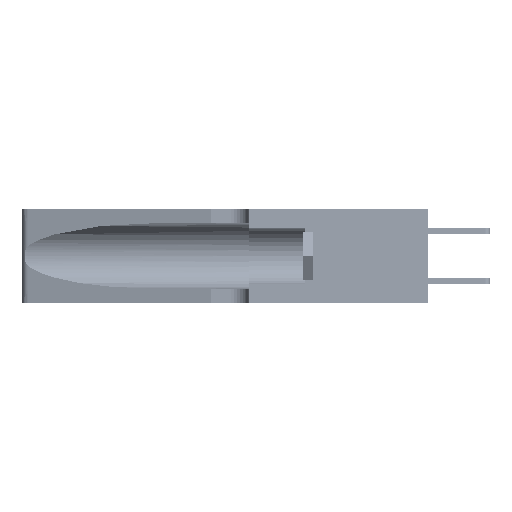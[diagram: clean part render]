
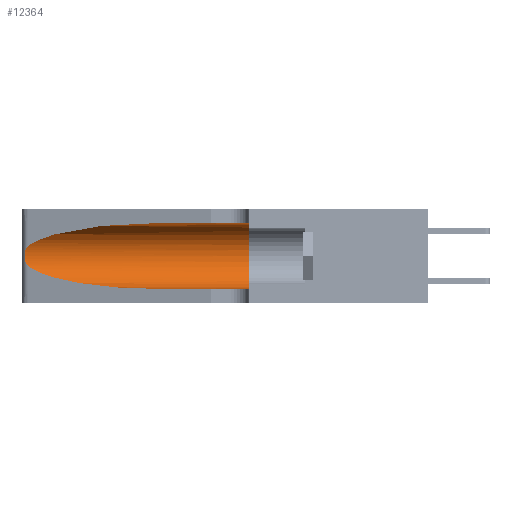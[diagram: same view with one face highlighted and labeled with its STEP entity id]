
A CAD part, left-side view. The second image highlights one B-rep face of the part: STEP entity #12364.
In plain terms, the highlighted cylindrical face has radius 3.308 mm (diameter 6.617 mm), a partial arc.
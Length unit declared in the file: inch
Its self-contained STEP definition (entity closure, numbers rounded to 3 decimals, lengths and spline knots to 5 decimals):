
#735 = CARTESIAN_POINT ( 'NONE',  ( 0.25856, 1.23593, 0.16098 ) ) ;
#1592 = CARTESIAN_POINT ( 'NONE',  ( 0.25487, 1.22718, 0.22369 ) ) ;
#2863 =( BOUNDED_CURVE ( )  B_SPLINE_CURVE ( 3, ( #27474, #7144, #24797, #3694 ),
 .UNSPECIFIED., .F., .F. ) 
 B_SPLINE_CURVE_WITH_KNOTS ( ( 4, 4 ),
 ( 3.44316, 4.71239 ),
 .UNSPECIFIED. ) 
 CURVE ( )  GEOMETRIC_REPRESENTATION_ITEM ( )  RATIONAL_B_SPLINE_CURVE ( ( 1., 0.87, 0.87, 1. ) ) 
 REPRESENTATION_ITEM ( '' )  );
#3694 = CARTESIAN_POINT ( 'NONE',  ( 0.1305, 0.72297, 0.05475 ) ) ;
#3899 = ORIENTED_EDGE ( 'NONE', *, *, #13138, .T. ) ;
#4337 = CARTESIAN_POINT ( 'NONE',  ( 0.1305, 0.35, 0.31525 ) ) ;
#5065 = ORIENTED_EDGE ( 'NONE', *, *, #23339, .T. ) ;
#6265 = DIRECTION ( 'NONE',  ( 0., -1., 0. ) ) ;
#7144 = CARTESIAN_POINT ( 'NONE',  ( 0.2373, 1.15595, 0.08982 ) ) ;
#7562 = DIRECTION ( 'NONE',  ( 0., 0., 1. ) ) ;
#8135 = FACE_OUTER_BOUND ( 'NONE', #32251, .T. ) ;
#8551 =( BOUNDED_CURVE ( )  B_SPLINE_CURVE ( 3, ( #12194, #26577, #44191, #1592 ),
 .UNSPECIFIED., .F., .F. ) 
 B_SPLINE_CURVE_WITH_KNOTS ( ( 4, 4 ),
 ( 1.5708, 2.84003 ),
 .UNSPECIFIED. ) 
 CURVE ( )  GEOMETRIC_REPRESENTATION_ITEM ( )  RATIONAL_B_SPLINE_CURVE ( ( 1., 0.87, 0.87, 1. ) ) 
 REPRESENTATION_ITEM ( '' )  );
#8889 = ORIENTED_EDGE ( 'NONE', *, *, #24045, .T. ) ;
#8992 = VERTEX_POINT ( 'NONE', #41970 ) ;
#9251 = VERTEX_POINT ( 'NONE', #41409 ) ;
#9920 = EDGE_CURVE ( 'NONE', #25475, #9251, #26015, .T. ) ;
#10131 = CARTESIAN_POINT ( 'NONE',  ( 0.1305, 1.61858, 0.05475 ) ) ;
#10462 = DIRECTION ( 'NONE',  ( 0., -1., 0. ) ) ;
#10898 = CYLINDRICAL_SURFACE ( 'NONE', #11148, 0.13025 ) ;
#11148 = AXIS2_PLACEMENT_3D ( 'NONE', #45881, #6265, #24544 ) ;
#11825 = CARTESIAN_POINT ( 'NONE',  ( 0.25487, 1.22718, 0.14631 ) ) ;
#12194 = CARTESIAN_POINT ( 'NONE',  ( 0.1305, 0.72297, 0.31525 ) ) ;
#12364 = ADVANCED_FACE ( 'NONE', ( #8135 ), #10898, .F. ) ;
#13138 = EDGE_CURVE ( 'NONE', #43283, #13946, #23740, .T. ) ;
#13278 = VECTOR ( 'NONE', #10462, 39.37008 ) ;
#13946 = VERTEX_POINT ( 'NONE', #33888 ) ;
#14356 = CARTESIAN_POINT ( 'NONE',  ( 0.26075, 1.23896, 0.178 ) ) ;
#14992 = LINE ( 'NONE', #10131, #13278 ) ;
#15132 = CARTESIAN_POINT ( 'NONE',  ( 0.25555, 1.22993, 0.14849 ) ) ;
#21440 = EDGE_CURVE ( 'NONE', #8992, #43283, #8551, .T. ) ;
#21520 = CARTESIAN_POINT ( 'NONE',  ( 0.1305, 1.61858, 0.31525 ) ) ;
#21534 = CARTESIAN_POINT ( 'NONE',  ( 0.26018, 1.23835, 0.19895 ) ) ;
#23339 = EDGE_CURVE ( 'NONE', #24796, #9251, #14992, .T. ) ;
#23740 = B_SPLINE_CURVE_WITH_KNOTS ( 'NONE', 3,
 ( #39850, #32170, #35783, #42957, #43236, #21534, #32016, #14356, #39389, #735, #29200, #36561, #15132, #11825 ),
 .UNSPECIFIED., .F., .F.,
 ( 4, 2, 2, 2, 2, 2, 4 ),
 ( 0., 0.00027, 0.00053, 0.00107, 0.0016, 0.00187, 0.00214 ),
 .UNSPECIFIED. ) ;
#24045 = EDGE_CURVE ( 'NONE', #13946, #24796, #2863, .T. ) ;
#24544 = DIRECTION ( 'NONE',  ( 0., 0., -1. ) ) ;
#24796 = VERTEX_POINT ( 'NONE', #28345 ) ;
#24797 = CARTESIAN_POINT ( 'NONE',  ( 0.18966, 0.96281, 0.05475 ) ) ;
#25475 = VERTEX_POINT ( 'NONE', #4337 ) ;
#25727 = ORIENTED_EDGE ( 'NONE', *, *, #42545, .F. ) ;
#26015 = CIRCLE ( 'NONE', #36586, 0.13025 ) ;
#26577 = CARTESIAN_POINT ( 'NONE',  ( 0.18966, 0.96281, 0.31525 ) ) ;
#27474 = CARTESIAN_POINT ( 'NONE',  ( 0.25487, 1.22718, 0.14631 ) ) ;
#27979 = ORIENTED_EDGE ( 'NONE', *, *, #21440, .T. ) ;
#28186 = CARTESIAN_POINT ( 'NONE',  ( 0.25487, 1.22718, 0.22369 ) ) ;
#28345 = CARTESIAN_POINT ( 'NONE',  ( 0.1305, 0.72297, 0.05475 ) ) ;
#29200 = CARTESIAN_POINT ( 'NONE',  ( 0.25789, 1.23486, 0.15765 ) ) ;
#31798 = CARTESIAN_POINT ( 'NONE',  ( 0.1305, 0.35, 0.185 ) ) ;
#32016 = CARTESIAN_POINT ( 'NONE',  ( 0.26075, 1.23896, 0.19203 ) ) ;
#32170 = CARTESIAN_POINT ( 'NONE',  ( 0.25555, 1.22994, 0.2215 ) ) ;
#32251 = EDGE_LOOP ( 'NONE', ( #27979, #3899, #8889, #5065, #39262, #25727 ) ) ;
#32783 = DIRECTION ( 'NONE',  ( 0., -1., 0. ) ) ;
#33034 = LINE ( 'NONE', #21520, #42520 ) ;
#33888 = CARTESIAN_POINT ( 'NONE',  ( 0.25487, 1.22718, 0.14631 ) ) ;
#35783 = CARTESIAN_POINT ( 'NONE',  ( 0.25639, 1.23184, 0.21858 ) ) ;
#36561 = CARTESIAN_POINT ( 'NONE',  ( 0.25639, 1.23186, 0.15144 ) ) ;
#36586 = AXIS2_PLACEMENT_3D ( 'NONE', #31798, #42874, #7562 ) ;
#39262 = ORIENTED_EDGE ( 'NONE', *, *, #9920, .F. ) ;
#39389 = CARTESIAN_POINT ( 'NONE',  ( 0.26017, 1.23833, 0.17102 ) ) ;
#39850 = CARTESIAN_POINT ( 'NONE',  ( 0.25487, 1.22718, 0.22369 ) ) ;
#41409 = CARTESIAN_POINT ( 'NONE',  ( 0.1305, 0.35, 0.05475 ) ) ;
#41970 = CARTESIAN_POINT ( 'NONE',  ( 0.1305, 0.72297, 0.31525 ) ) ;
#42520 = VECTOR ( 'NONE', #32783, 39.37008 ) ;
#42545 = EDGE_CURVE ( 'NONE', #8992, #25475, #33034, .T. ) ;
#42874 = DIRECTION ( 'NONE',  ( 0., 1., 0. ) ) ;
#42957 = CARTESIAN_POINT ( 'NONE',  ( 0.25787, 1.23484, 0.2124 ) ) ;
#43236 = CARTESIAN_POINT ( 'NONE',  ( 0.25854, 1.2359, 0.20912 ) ) ;
#43283 = VERTEX_POINT ( 'NONE', #28186 ) ;
#44191 = CARTESIAN_POINT ( 'NONE',  ( 0.2373, 1.15595, 0.28018 ) ) ;
#45881 = CARTESIAN_POINT ( 'NONE',  ( 0.1305, 1.61858, 0.185 ) ) ;
